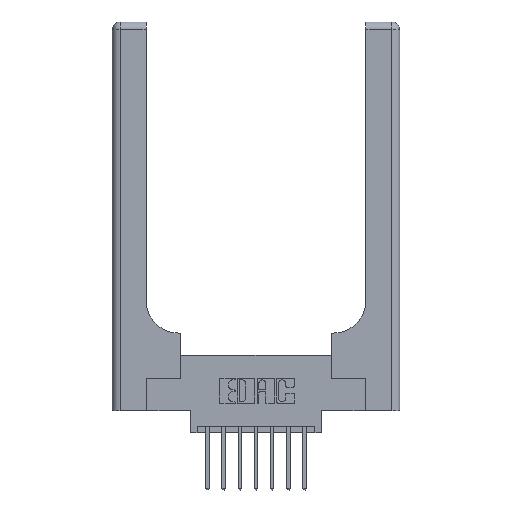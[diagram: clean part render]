
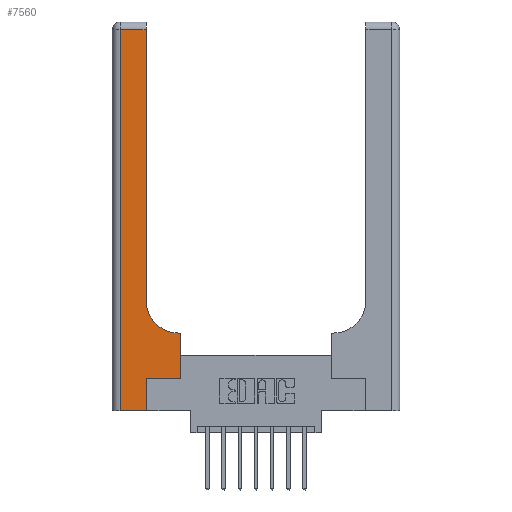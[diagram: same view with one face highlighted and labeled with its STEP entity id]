
A CAD part, top view. The second image highlights one B-rep face of the part: STEP entity #7560.
In plain terms, the highlighted planar face has unit normal (0, 0, 1).
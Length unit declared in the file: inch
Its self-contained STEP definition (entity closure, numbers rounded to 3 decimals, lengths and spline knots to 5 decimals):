
#272 = VERTEX_POINT ( 'NONE', #11512 ) ;
#415 = CARTESIAN_POINT ( 'NONE',  ( 0.265, 0., 0.37 ) ) ;
#496 = LINE ( 'NONE', #13195, #2279 ) ;
#531 = EDGE_CURVE ( 'NONE', #9466, #272, #5937, .T. ) ;
#950 = CARTESIAN_POINT ( 'NONE',  ( 0.265, 0.25, 0.37 ) ) ;
#1615 = DIRECTION ( 'NONE',  ( 0., 0., -1. ) ) ;
#1643 = VERTEX_POINT ( 'NONE', #5037 ) ;
#2034 = LINE ( 'NONE', #11175, #12580 ) ;
#2120 = LINE ( 'NONE', #7932, #3614 ) ;
#2279 = VECTOR ( 'NONE', #5044, 39.37008 ) ;
#2348 = EDGE_CURVE ( 'NONE', #272, #4943, #2120, .T. ) ;
#2406 = CARTESIAN_POINT ( 'NONE',  ( 0., 2.94, 0.37 ) ) ;
#2426 = ORIENTED_EDGE ( 'NONE', *, *, #14141, .T. ) ;
#2604 = ORIENTED_EDGE ( 'NONE', *, *, #531, .T. ) ;
#2742 = CARTESIAN_POINT ( 'NONE',  ( 0., 3., 0.37 ) ) ;
#2909 = CARTESIAN_POINT ( 'NONE',  ( 0.51, 0.85, 0.37 ) ) ;
#3190 = CARTESIAN_POINT ( 'NONE',  ( 0.26, 0.6, 0.37 ) ) ;
#3288 = EDGE_CURVE ( 'NONE', #11753, #5843, #2034, .T. ) ;
#3495 = CARTESIAN_POINT ( 'NONE',  ( 0.06, 0., 0.37 ) ) ;
#3614 = VECTOR ( 'NONE', #12262, 39.37008 ) ;
#3791 = CARTESIAN_POINT ( 'NONE',  ( 0.528, 0.25, 0.37 ) ) ;
#3893 = LINE ( 'NONE', #9512, #9547 ) ;
#3967 = DIRECTION ( 'NONE',  ( 0., -1., 0. ) ) ;
#4063 = CARTESIAN_POINT ( 'NONE',  ( 0.26, 2.94, 0.37 ) ) ;
#4305 = ORIENTED_EDGE ( 'NONE', *, *, #9321, .T. ) ;
#4317 = DIRECTION ( 'NONE',  ( -1., 0., 0. ) ) ;
#4387 = VECTOR ( 'NONE', #7058, 39.37008 ) ;
#4581 = CARTESIAN_POINT ( 'NONE',  ( 0., 0., 0.37 ) ) ;
#4903 = ORIENTED_EDGE ( 'NONE', *, *, #11212, .T. ) ;
#4943 = VERTEX_POINT ( 'NONE', #4063 ) ;
#5037 = CARTESIAN_POINT ( 'NONE',  ( 0.06, 2.94, 0.37 ) ) ;
#5044 = DIRECTION ( 'NONE',  ( 0., 1., 0. ) ) ;
#5066 = VERTEX_POINT ( 'NONE', #415 ) ;
#5190 = CARTESIAN_POINT ( 'NONE',  ( 0.265, 0.25, 0.37 ) ) ;
#5484 = VERTEX_POINT ( 'NONE', #5190 ) ;
#5774 = VERTEX_POINT ( 'NONE', #3495 ) ;
#5843 = VERTEX_POINT ( 'NONE', #10724 ) ;
#5937 = CIRCLE ( 'NONE', #8373, 0.25 ) ;
#6183 = FACE_OUTER_BOUND ( 'NONE', #14848, .T. ) ;
#6790 = VECTOR ( 'NONE', #11805, 39.37008 ) ;
#6823 = DIRECTION ( 'NONE',  ( 0., 1., 0. ) ) ;
#6880 = LINE ( 'NONE', #4581, #6790 ) ;
#7058 = DIRECTION ( 'NONE',  ( -1., 0., 0. ) ) ;
#7484 = DIRECTION ( 'NONE',  ( -1., 0., 0. ) ) ;
#7560 = ADVANCED_FACE ( 'NONE', ( #6183 ), #13408, .F. ) ;
#7932 = CARTESIAN_POINT ( 'NONE',  ( 0.26, 3., 0.37 ) ) ;
#8140 = LINE ( 'NONE', #3190, #13702 ) ;
#8373 = AXIS2_PLACEMENT_3D ( 'NONE', #2909, #10747, #11061 ) ;
#8676 = AXIS2_PLACEMENT_3D ( 'NONE', #2742, #1615, #7484 ) ;
#9191 = ORIENTED_EDGE ( 'NONE', *, *, #2348, .T. ) ;
#9321 = EDGE_CURVE ( 'NONE', #4943, #1643, #12834, .T. ) ;
#9466 = VERTEX_POINT ( 'NONE', #11660 ) ;
#9512 = CARTESIAN_POINT ( 'NONE',  ( 0.06, 3., 0.37 ) ) ;
#9547 = VECTOR ( 'NONE', #3967, 39.37008 ) ;
#10094 = ORIENTED_EDGE ( 'NONE', *, *, #12292, .T. ) ;
#10724 = CARTESIAN_POINT ( 'NONE',  ( 0.528, 0.6, 0.37 ) ) ;
#10747 = DIRECTION ( 'NONE',  ( 0., 0., -1. ) ) ;
#10951 = ORIENTED_EDGE ( 'NONE', *, *, #13709, .T. ) ;
#11061 = DIRECTION ( 'NONE',  ( 1., 0., 0. ) ) ;
#11175 = CARTESIAN_POINT ( 'NONE',  ( 0.528, 0.25, 0.37 ) ) ;
#11212 = EDGE_CURVE ( 'NONE', #5774, #5066, #6880, .T. ) ;
#11485 = ORIENTED_EDGE ( 'NONE', *, *, #3288, .T. ) ;
#11512 = CARTESIAN_POINT ( 'NONE',  ( 0.26, 0.85, 0.37 ) ) ;
#11660 = CARTESIAN_POINT ( 'NONE',  ( 0.51, 0.6, 0.37 ) ) ;
#11753 = VERTEX_POINT ( 'NONE', #3791 ) ;
#11805 = DIRECTION ( 'NONE',  ( 1., 0., 0. ) ) ;
#12262 = DIRECTION ( 'NONE',  ( 0., 1., 0. ) ) ;
#12292 = EDGE_CURVE ( 'NONE', #5484, #11753, #14515, .T. ) ;
#12459 = VECTOR ( 'NONE', #13585, 39.37008 ) ;
#12580 = VECTOR ( 'NONE', #6823, 39.37008 ) ;
#12834 = LINE ( 'NONE', #2406, #4387 ) ;
#12958 = ORIENTED_EDGE ( 'NONE', *, *, #13280, .T. ) ;
#13195 = CARTESIAN_POINT ( 'NONE',  ( 0.265, 0., 0.37 ) ) ;
#13280 = EDGE_CURVE ( 'NONE', #5843, #9466, #8140, .T. ) ;
#13408 = PLANE ( 'NONE',  #8676 ) ;
#13585 = DIRECTION ( 'NONE',  ( 1., 0., 0. ) ) ;
#13702 = VECTOR ( 'NONE', #4317, 39.37008 ) ;
#13709 = EDGE_CURVE ( 'NONE', #5066, #5484, #496, .T. ) ;
#14141 = EDGE_CURVE ( 'NONE', #1643, #5774, #3893, .T. ) ;
#14515 = LINE ( 'NONE', #950, #12459 ) ;
#14848 = EDGE_LOOP ( 'NONE', ( #9191, #4305, #2426, #4903, #10951, #10094, #11485, #12958, #2604 ) ) ;
